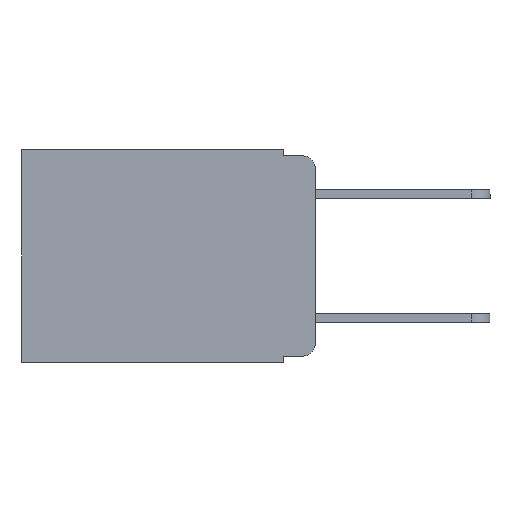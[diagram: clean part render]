
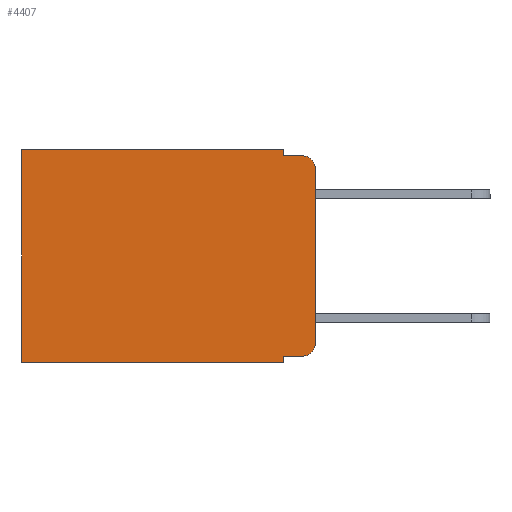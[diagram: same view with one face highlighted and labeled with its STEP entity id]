
A CAD part, left-side view. The second image highlights one B-rep face of the part: STEP entity #4407.
In plain terms, the highlighted planar face has unit normal (-1, 0, 0).
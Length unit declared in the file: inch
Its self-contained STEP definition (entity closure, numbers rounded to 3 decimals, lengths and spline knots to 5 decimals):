
#201 = EDGE_CURVE ( 'NONE', #7463, #2016, #4444, .T. ) ;
#509 = EDGE_CURVE ( 'NONE', #1119, #6053, #2985, .T. ) ;
#512 = VERTEX_POINT ( 'NONE', #9097 ) ;
#835 = CARTESIAN_POINT ( 'NONE',  ( 0.298, 0.02, -0.313 ) ) ;
#964 = VERTEX_POINT ( 'NONE', #8303 ) ;
#1106 = VERTEX_POINT ( 'NONE', #3409 ) ;
#1119 = VERTEX_POINT ( 'NONE', #5704 ) ;
#1346 = LINE ( 'NONE', #8817, #3747 ) ;
#1484 = VECTOR ( 'NONE', #8106, 39.37008 ) ;
#1661 = CARTESIAN_POINT ( 'NONE',  ( 0.298, 0.051, 0. ) ) ;
#1699 = CARTESIAN_POINT ( 'NONE',  ( 0.298, 0.051, -0.333 ) ) ;
#1735 = ORIENTED_EDGE ( 'NONE', *, *, #509, .T. ) ;
#1886 = VECTOR ( 'NONE', #3010, 39.37008 ) ;
#1912 = VERTEX_POINT ( 'NONE', #8475 ) ;
#1961 = DIRECTION ( 'NONE',  ( 0., -1., 0. ) ) ;
#1966 = LINE ( 'NONE', #2250, #5962 ) ;
#2016 = VERTEX_POINT ( 'NONE', #4564 ) ;
#2096 = EDGE_CURVE ( 'NONE', #964, #2545, #4138, .T. ) ;
#2250 = CARTESIAN_POINT ( 'NONE',  ( 0.298, 0.051, -0.333 ) ) ;
#2363 = ORIENTED_EDGE ( 'NONE', *, *, #6081, .F. ) ;
#2545 = VERTEX_POINT ( 'NONE', #3317 ) ;
#2560 = EDGE_CURVE ( 'NONE', #2545, #1106, #8750, .T. ) ;
#2631 = EDGE_CURVE ( 'NONE', #512, #2016, #4006, .T. ) ;
#2670 = ORIENTED_EDGE ( 'NONE', *, *, #2560, .F. ) ;
#2790 = ORIENTED_EDGE ( 'NONE', *, *, #4776, .F. ) ;
#2884 = ORIENTED_EDGE ( 'NONE', *, *, #201, .F. ) ;
#2899 = DIRECTION ( 'NONE',  ( -1., 0., 0. ) ) ;
#2910 = ORIENTED_EDGE ( 'NONE', *, *, #2631, .T. ) ;
#2985 = CIRCLE ( 'NONE', #7416, 0.02 ) ;
#3010 = DIRECTION ( 'NONE',  ( 0., 0., -1. ) ) ;
#3085 = VECTOR ( 'NONE', #3235, 39.37008 ) ;
#3099 = CARTESIAN_POINT ( 'NONE',  ( 0.298, 0., -0.313 ) ) ;
#3147 = ORIENTED_EDGE ( 'NONE', *, *, #3210, .T. ) ;
#3178 = CARTESIAN_POINT ( 'NONE',  ( 0.298, 0.051, -0.343 ) ) ;
#3210 = EDGE_CURVE ( 'NONE', #3291, #1119, #1966, .T. ) ;
#3235 = DIRECTION ( 'NONE',  ( 0., 0., -1. ) ) ;
#3291 = VERTEX_POINT ( 'NONE', #1699 ) ;
#3317 = CARTESIAN_POINT ( 'NONE',  ( 0.298, 0.051, -0.01 ) ) ;
#3396 = DIRECTION ( 'NONE',  ( 0., 0., -1. ) ) ;
#3409 = CARTESIAN_POINT ( 'NONE',  ( 0.298, 0.02, -0.01 ) ) ;
#3747 = VECTOR ( 'NONE', #8814, 39.37008 ) ;
#3774 = ORIENTED_EDGE ( 'NONE', *, *, #2096, .F. ) ;
#3794 = ORIENTED_EDGE ( 'NONE', *, *, #4055, .T. ) ;
#3857 = LINE ( 'NONE', #8101, #1484 ) ;
#4006 = LINE ( 'NONE', #5558, #5992 ) ;
#4055 = EDGE_CURVE ( 'NONE', #964, #512, #3857, .T. ) ;
#4138 = LINE ( 'NONE', #1661, #1886 ) ;
#4338 = CARTESIAN_POINT ( 'NONE',  ( 0.298, 0., 0. ) ) ;
#4407 = ADVANCED_FACE ( 'NONE', ( #6346 ), #5743, .F. ) ;
#4444 = LINE ( 'NONE', #7713, #5988 ) ;
#4564 = CARTESIAN_POINT ( 'NONE',  ( 0.298, 0.473, -0.343 ) ) ;
#4776 = EDGE_CURVE ( 'NONE', #3291, #7463, #1346, .T. ) ;
#4940 = EDGE_LOOP ( 'NONE', ( #2363, #6202, #2670, #3774, #3794, #2910, #2884, #2790, #3147, #1735 ) ) ;
#5406 = AXIS2_PLACEMENT_3D ( 'NONE', #4338, #7507, #3396 ) ;
#5558 = CARTESIAN_POINT ( 'NONE',  ( 0.298, 0.473, 0. ) ) ;
#5704 = CARTESIAN_POINT ( 'NONE',  ( 0.298, 0.02, -0.333 ) ) ;
#5743 = PLANE ( 'NONE',  #5406 ) ;
#5934 = CARTESIAN_POINT ( 'NONE',  ( 0.298, 0.051, -0.01 ) ) ;
#5962 = VECTOR ( 'NONE', #1961, 39.37008 ) ;
#5988 = VECTOR ( 'NONE', #7862, 39.37008 ) ;
#5992 = VECTOR ( 'NONE', #8941, 39.37008 ) ;
#6053 = VERTEX_POINT ( 'NONE', #3099 ) ;
#6081 = EDGE_CURVE ( 'NONE', #1912, #6053, #8184, .T. ) ;
#6202 = ORIENTED_EDGE ( 'NONE', *, *, #6230, .T. ) ;
#6230 = EDGE_CURVE ( 'NONE', #1912, #1106, #6959, .T. ) ;
#6346 = FACE_OUTER_BOUND ( 'NONE', #4940, .T. ) ;
#6580 = CARTESIAN_POINT ( 'NONE',  ( 0.298, 0.02, -0.03 ) ) ;
#6657 = AXIS2_PLACEMENT_3D ( 'NONE', #6580, #2899, #7224 ) ;
#6959 = CIRCLE ( 'NONE', #6657, 0.02 ) ;
#7094 = VECTOR ( 'NONE', #8189, 39.37008 ) ;
#7120 = CARTESIAN_POINT ( 'NONE',  ( 0.298, 0., 0. ) ) ;
#7224 = DIRECTION ( 'NONE',  ( 0., 0., -1. ) ) ;
#7416 = AXIS2_PLACEMENT_3D ( 'NONE', #835, #8763, #8764 ) ;
#7463 = VERTEX_POINT ( 'NONE', #3178 ) ;
#7507 = DIRECTION ( 'NONE',  ( 1., 0., 0. ) ) ;
#7713 = CARTESIAN_POINT ( 'NONE',  ( 0.298, 0., -0.343 ) ) ;
#7862 = DIRECTION ( 'NONE',  ( 0., 1., 0. ) ) ;
#8101 = CARTESIAN_POINT ( 'NONE',  ( 0.298, 0., 0. ) ) ;
#8106 = DIRECTION ( 'NONE',  ( 0., 1., 0. ) ) ;
#8184 = LINE ( 'NONE', #7120, #3085 ) ;
#8189 = DIRECTION ( 'NONE',  ( 0., -1., 0. ) ) ;
#8303 = CARTESIAN_POINT ( 'NONE',  ( 0.298, 0.051, 0. ) ) ;
#8475 = CARTESIAN_POINT ( 'NONE',  ( 0.298, 0., -0.03 ) ) ;
#8750 = LINE ( 'NONE', #5934, #7094 ) ;
#8763 = DIRECTION ( 'NONE',  ( -1., 0., 0. ) ) ;
#8764 = DIRECTION ( 'NONE',  ( 0., 0., -1. ) ) ;
#8814 = DIRECTION ( 'NONE',  ( 0., 0., -1. ) ) ;
#8817 = CARTESIAN_POINT ( 'NONE',  ( 0.298, 0.051, 0. ) ) ;
#8941 = DIRECTION ( 'NONE',  ( 0., 0., -1. ) ) ;
#9097 = CARTESIAN_POINT ( 'NONE',  ( 0.298, 0.473, 0. ) ) ;
